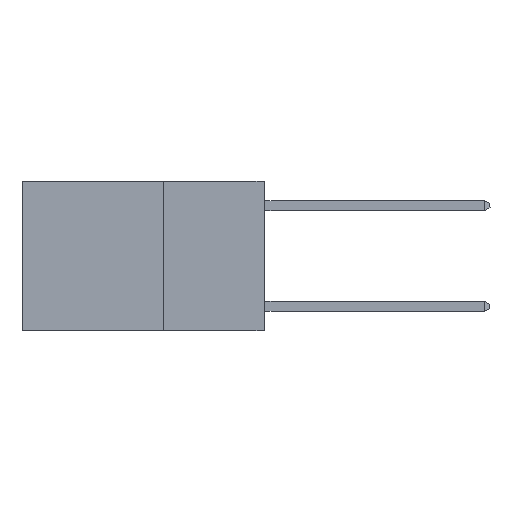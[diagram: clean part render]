
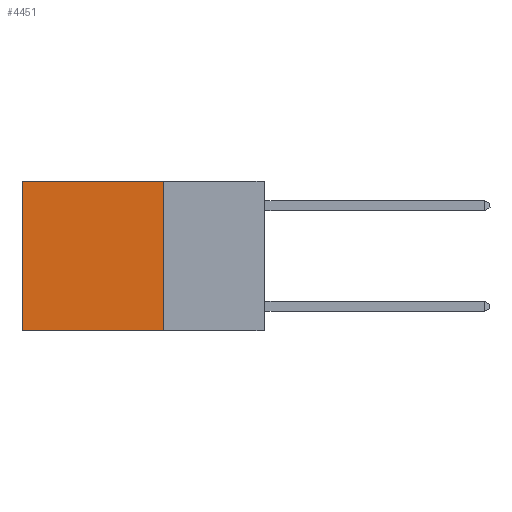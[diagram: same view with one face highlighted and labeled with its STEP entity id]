
A CAD part, left-side view. The second image highlights one B-rep face of the part: STEP entity #4451.
In plain terms, the highlighted planar face has unit normal (-1, 0, 0).
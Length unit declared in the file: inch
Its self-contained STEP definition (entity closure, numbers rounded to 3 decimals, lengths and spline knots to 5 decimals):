
#133 = DIRECTION ( 'NONE',  ( 0., 1., 0. ) ) ;
#165 = VECTOR ( 'NONE', #3763, 39.37008 ) ;
#1243 = CARTESIAN_POINT ( 'NONE',  ( 0.2625, 0.25, -0.37 ) ) ;
#1410 = EDGE_CURVE ( 'NONE', #9161, #2679, #4884, .T. ) ;
#1466 = CARTESIAN_POINT ( 'NONE',  ( 0.2625, 0.25, -0.37 ) ) ;
#1785 = DIRECTION ( 'NONE',  ( 0., 0., -1. ) ) ;
#1860 = DIRECTION ( 'NONE',  ( 1., 0., 0. ) ) ;
#1993 = ORIENTED_EDGE ( 'NONE', *, *, #5465, .T. ) ;
#2299 = FACE_OUTER_BOUND ( 'NONE', #4227, .T. ) ;
#2393 = CARTESIAN_POINT ( 'NONE',  ( 0.2625, 0.25, 0. ) ) ;
#2457 = ORIENTED_EDGE ( 'NONE', *, *, #5517, .F. ) ;
#2679 = VERTEX_POINT ( 'NONE', #3389 ) ;
#2700 = AXIS2_PLACEMENT_3D ( 'NONE', #9731, #1860, #1785 ) ;
#2744 = VECTOR ( 'NONE', #133, 39.37008 ) ;
#2840 = VERTEX_POINT ( 'NONE', #1243 ) ;
#3157 = DIRECTION ( 'NONE',  ( 0., 1., 0. ) ) ;
#3314 = VERTEX_POINT ( 'NONE', #10254 ) ;
#3389 = CARTESIAN_POINT ( 'NONE',  ( 0.2625, 0.6, 0. ) ) ;
#3763 = DIRECTION ( 'NONE',  ( 0., 0., -1. ) ) ;
#3817 = DIRECTION ( 'NONE',  ( 0., 0., -1. ) ) ;
#4227 = EDGE_LOOP ( 'NONE', ( #1993, #2457, #6753, #5198 ) ) ;
#4399 = VECTOR ( 'NONE', #3157, 39.37008 ) ;
#4451 = ADVANCED_FACE ( 'NONE', ( #2299 ), #7375, .F. ) ;
#4884 = LINE ( 'NONE', #6870, #2744 ) ;
#5198 = ORIENTED_EDGE ( 'NONE', *, *, #1410, .T. ) ;
#5465 = EDGE_CURVE ( 'NONE', #2679, #3314, #6882, .T. ) ;
#5517 = EDGE_CURVE ( 'NONE', #2840, #3314, #6640, .T. ) ;
#6640 = LINE ( 'NONE', #1466, #4399 ) ;
#6753 = ORIENTED_EDGE ( 'NONE', *, *, #10303, .F. ) ;
#6870 = CARTESIAN_POINT ( 'NONE',  ( 0.2625, 0.25, 0. ) ) ;
#6882 = LINE ( 'NONE', #7660, #8526 ) ;
#7375 = PLANE ( 'NONE',  #2700 ) ;
#7660 = CARTESIAN_POINT ( 'NONE',  ( 0.2625, 0.6, 0. ) ) ;
#8526 = VECTOR ( 'NONE', #3817, 39.37008 ) ;
#9161 = VERTEX_POINT ( 'NONE', #2393 ) ;
#9731 = CARTESIAN_POINT ( 'NONE',  ( 0.2625, 0.25, 0. ) ) ;
#10026 = CARTESIAN_POINT ( 'NONE',  ( 0.2625, 0.25, 0. ) ) ;
#10034 = LINE ( 'NONE', #10026, #165 ) ;
#10254 = CARTESIAN_POINT ( 'NONE',  ( 0.2625, 0.6, -0.37 ) ) ;
#10303 = EDGE_CURVE ( 'NONE', #9161, #2840, #10034, .T. ) ;
